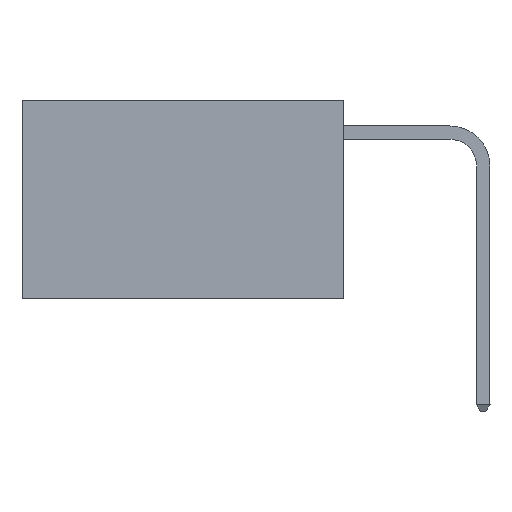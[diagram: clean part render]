
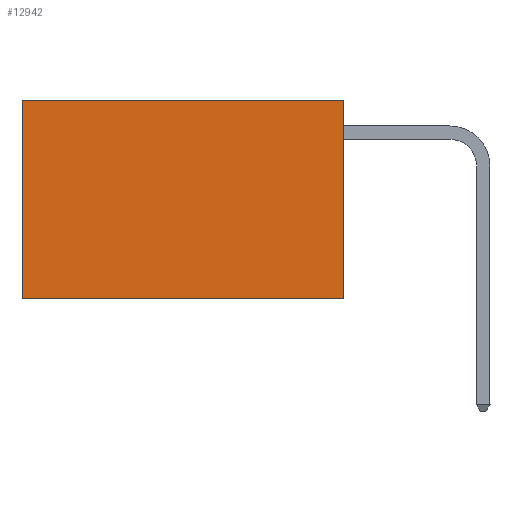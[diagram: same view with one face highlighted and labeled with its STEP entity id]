
A CAD part, left-side view. The second image highlights one B-rep face of the part: STEP entity #12942.
In plain terms, the highlighted planar face has unit normal (-1, 0, 0).
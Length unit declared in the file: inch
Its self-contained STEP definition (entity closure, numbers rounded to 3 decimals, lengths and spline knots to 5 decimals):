
#20 = CARTESIAN_POINT ( 'NONE',  ( 0.2625, 0., 0. ) ) ;
#993 = EDGE_LOOP ( 'NONE', ( #1628, #3323, #12410, #14031 ) ) ;
#1409 = DIRECTION ( 'NONE',  ( 1., 0., 0. ) ) ;
#1628 = ORIENTED_EDGE ( 'NONE', *, *, #9849, .T. ) ;
#3323 = ORIENTED_EDGE ( 'NONE', *, *, #11018, .F. ) ;
#3970 = EDGE_CURVE ( 'NONE', #7342, #5742, #4425, .T. ) ;
#4425 = LINE ( 'NONE', #15796, #10829 ) ;
#4566 = VERTEX_POINT ( 'NONE', #12518 ) ;
#4802 = DIRECTION ( 'NONE',  ( 0., 0., -1. ) ) ;
#5406 = CARTESIAN_POINT ( 'NONE',  ( 0.2625, 0.6, 0. ) ) ;
#5540 = VECTOR ( 'NONE', #13870, 39.37008 ) ;
#5742 = VERTEX_POINT ( 'NONE', #5406 ) ;
#6810 = EDGE_CURVE ( 'NONE', #7342, #4566, #10786, .T. ) ;
#7342 = VERTEX_POINT ( 'NONE', #8234 ) ;
#7429 = VECTOR ( 'NONE', #4802, 39.37008 ) ;
#7966 = PLANE ( 'NONE',  #14633 ) ;
#8234 = CARTESIAN_POINT ( 'NONE',  ( 0.2625, 0., 0. ) ) ;
#8534 = LINE ( 'NONE', #16410, #5540 ) ;
#8624 = CARTESIAN_POINT ( 'NONE',  ( 0.2625, 0., 0. ) ) ;
#8882 = DIRECTION ( 'NONE',  ( 0., 1., 0. ) ) ;
#9106 = DIRECTION ( 'NONE',  ( 0., 1., 0. ) ) ;
#9849 = EDGE_CURVE ( 'NONE', #5742, #12040, #8534, .T. ) ;
#9904 = CARTESIAN_POINT ( 'NONE',  ( 0.2625, 0.6, -0.37 ) ) ;
#10200 = FACE_OUTER_BOUND ( 'NONE', #993, .T. ) ;
#10492 = DIRECTION ( 'NONE',  ( 0., 0., -1. ) ) ;
#10786 = LINE ( 'NONE', #8624, #7429 ) ;
#10829 = VECTOR ( 'NONE', #9106, 39.37008 ) ;
#11018 = EDGE_CURVE ( 'NONE', #4566, #12040, #15905, .T. ) ;
#12040 = VERTEX_POINT ( 'NONE', #9904 ) ;
#12410 = ORIENTED_EDGE ( 'NONE', *, *, #6810, .F. ) ;
#12512 = VECTOR ( 'NONE', #8882, 39.37008 ) ;
#12518 = CARTESIAN_POINT ( 'NONE',  ( 0.2625, 0., -0.37 ) ) ;
#12942 = ADVANCED_FACE ( 'NONE', ( #10200 ), #7966, .F. ) ;
#13870 = DIRECTION ( 'NONE',  ( 0., 0., -1. ) ) ;
#14031 = ORIENTED_EDGE ( 'NONE', *, *, #3970, .T. ) ;
#14633 = AXIS2_PLACEMENT_3D ( 'NONE', #20, #1409, #10492 ) ;
#15796 = CARTESIAN_POINT ( 'NONE',  ( 0.2625, 0., 0. ) ) ;
#15905 = LINE ( 'NONE', #16557, #12512 ) ;
#16410 = CARTESIAN_POINT ( 'NONE',  ( 0.2625, 0.6, 0. ) ) ;
#16557 = CARTESIAN_POINT ( 'NONE',  ( 0.2625, 0., -0.37 ) ) ;
